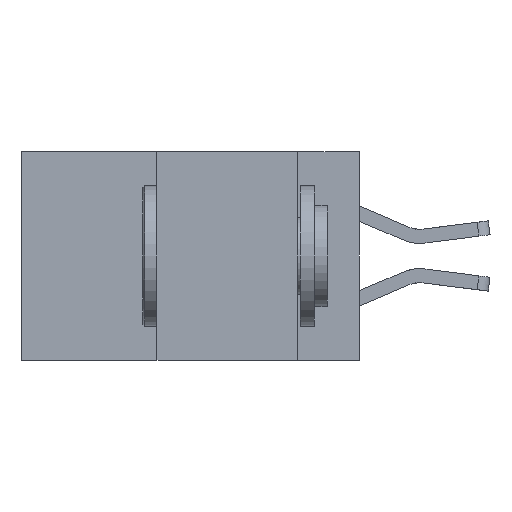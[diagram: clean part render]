
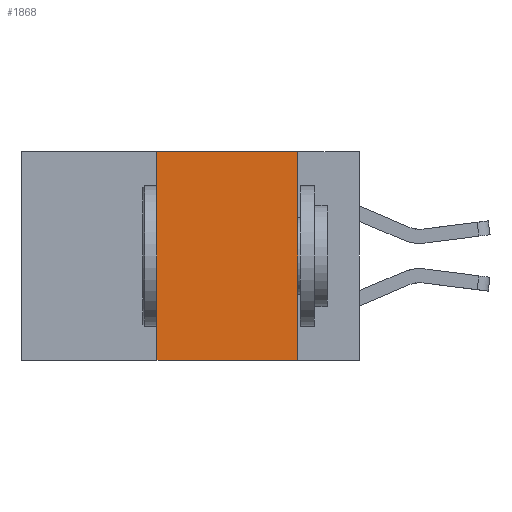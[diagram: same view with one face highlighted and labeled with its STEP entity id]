
A CAD part, left-side view. The second image highlights one B-rep face of the part: STEP entity #1868.
In plain terms, the highlighted planar face has unit normal (-1, 0, 0).
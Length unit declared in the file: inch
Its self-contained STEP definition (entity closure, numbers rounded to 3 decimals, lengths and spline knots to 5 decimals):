
#873 = LINE ( 'NONE', #3231, #6819 ) ;
#1868 = ADVANCED_FACE ( 'NONE', ( #9124 ), #11400, .F. ) ;
#2067 = ORIENTED_EDGE ( 'NONE', *, *, #7140, .F. ) ;
#2225 = ORIENTED_EDGE ( 'NONE', *, *, #5839, .F. ) ;
#2783 = DIRECTION ( 'NONE',  ( 0., -1., 0. ) ) ;
#3231 = CARTESIAN_POINT ( 'NONE',  ( 0., 0.6, -0.37 ) ) ;
#4252 = VERTEX_POINT ( 'NONE', #9255 ) ;
#4341 = ORIENTED_EDGE ( 'NONE', *, *, #9270, .F. ) ;
#4477 = DIRECTION ( 'NONE',  ( 0., 0., 1. ) ) ;
#4870 = VERTEX_POINT ( 'NONE', #11273 ) ;
#4959 = CARTESIAN_POINT ( 'NONE',  ( 0., 0.36, -0.37 ) ) ;
#5211 = DIRECTION ( 'NONE',  ( 0., 0., -1. ) ) ;
#5839 = EDGE_CURVE ( 'NONE', #4870, #7634, #9791, .T. ) ;
#5934 = VECTOR ( 'NONE', #5211, 39.37008 ) ;
#6279 = CARTESIAN_POINT ( 'NONE',  ( 0., 0.6, 0. ) ) ;
#6770 = VECTOR ( 'NONE', #4477, 39.37008 ) ;
#6819 = VECTOR ( 'NONE', #7718, 39.37008 ) ;
#6830 = ORIENTED_EDGE ( 'NONE', *, *, #11324, .T. ) ;
#7140 = EDGE_CURVE ( 'NONE', #7634, #4252, #9098, .T. ) ;
#7634 = VERTEX_POINT ( 'NONE', #13061 ) ;
#7718 = DIRECTION ( 'NONE',  ( 0., -1., 0. ) ) ;
#9098 = LINE ( 'NONE', #10576, #5934 ) ;
#9124 = FACE_OUTER_BOUND ( 'NONE', #10823, .T. ) ;
#9255 = CARTESIAN_POINT ( 'NONE',  ( 0., 0.11, -0.37 ) ) ;
#9270 = EDGE_CURVE ( 'NONE', #12891, #4870, #9578, .T. ) ;
#9578 = LINE ( 'NONE', #12106, #6770 ) ;
#9791 = LINE ( 'NONE', #6279, #11998 ) ;
#10576 = CARTESIAN_POINT ( 'NONE',  ( 0., 0.11, 0. ) ) ;
#10823 = EDGE_LOOP ( 'NONE', ( #2067, #2225, #4341, #6830 ) ) ;
#11273 = CARTESIAN_POINT ( 'NONE',  ( 0., 0.36, 0. ) ) ;
#11291 = AXIS2_PLACEMENT_3D ( 'NONE', #11323, #11322, #11296 ) ;
#11296 = DIRECTION ( 'NONE',  ( 0., 0., -1. ) ) ;
#11322 = DIRECTION ( 'NONE',  ( 1., 0., 0. ) ) ;
#11324 = EDGE_CURVE ( 'NONE', #12891, #4252, #873, .T. ) ;
#11323 = CARTESIAN_POINT ( 'NONE',  ( 0., 0.6, 0. ) ) ;
#11400 = PLANE ( 'NONE',  #11291 ) ;
#11998 = VECTOR ( 'NONE', #2783, 39.37008 ) ;
#12106 = CARTESIAN_POINT ( 'NONE',  ( 0., 0.36, 0. ) ) ;
#12891 = VERTEX_POINT ( 'NONE', #4959 ) ;
#13061 = CARTESIAN_POINT ( 'NONE',  ( 0., 0.11, 0. ) ) ;
